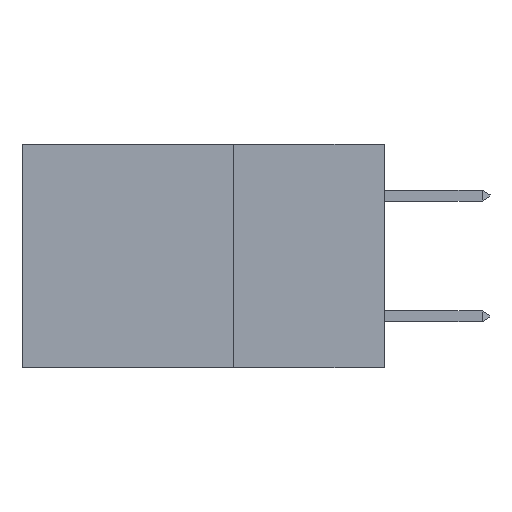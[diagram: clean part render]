
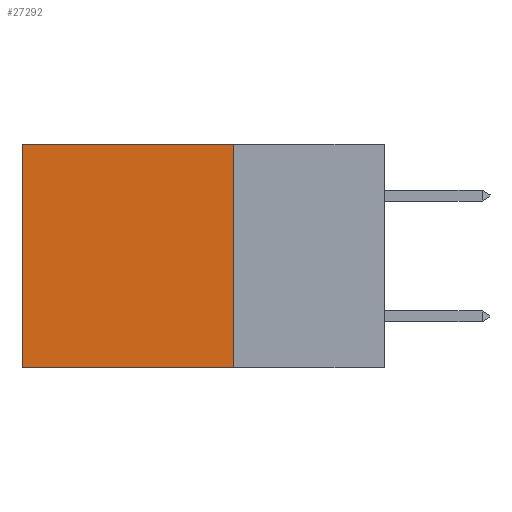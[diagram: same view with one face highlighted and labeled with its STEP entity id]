
A CAD part, left-side view. The second image highlights one B-rep face of the part: STEP entity #27292.
In plain terms, the highlighted planar face has unit normal (-1, 0, 0).
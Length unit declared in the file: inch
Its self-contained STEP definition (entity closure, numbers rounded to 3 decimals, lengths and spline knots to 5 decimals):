
#232 = EDGE_CURVE ( 'NONE', #1115, #25379, #8857, .T. ) ;
#1115 = VERTEX_POINT ( 'NONE', #8701 ) ;
#1706 = DIRECTION ( 'NONE',  ( 0., 0., -1. ) ) ;
#2444 = ORIENTED_EDGE ( 'NONE', *, *, #23544, .F. ) ;
#2747 = CARTESIAN_POINT ( 'NONE',  ( 0.2875, 0.25, -0.37 ) ) ;
#4359 = CARTESIAN_POINT ( 'NONE',  ( 0.2875, 0.25, 0. ) ) ;
#5426 = VERTEX_POINT ( 'NONE', #18399 ) ;
#8701 = CARTESIAN_POINT ( 'NONE',  ( 0.2875, 0.6, 0. ) ) ;
#8857 = LINE ( 'NONE', #19627, #31252 ) ;
#9338 = DIRECTION ( 'NONE',  ( 1., 0., 0. ) ) ;
#9750 = VECTOR ( 'NONE', #28491, 39.37008 ) ;
#13326 = ORIENTED_EDGE ( 'NONE', *, *, #232, .T. ) ;
#13913 = DIRECTION ( 'NONE',  ( 0., 1., 0. ) ) ;
#15936 = EDGE_LOOP ( 'NONE', ( #13326, #2444, #22675, #24786 ) ) ;
#16980 = LINE ( 'NONE', #4359, #9750 ) ;
#18399 = CARTESIAN_POINT ( 'NONE',  ( 0.2875, 0.25, 0. ) ) ;
#19078 = EDGE_CURVE ( 'NONE', #5426, #1115, #28894, .T. ) ;
#19394 = DIRECTION ( 'NONE',  ( 0., 0., -1. ) ) ;
#19627 = CARTESIAN_POINT ( 'NONE',  ( 0.2875, 0.6, 0. ) ) ;
#20746 = EDGE_CURVE ( 'NONE', #5426, #29613, #16980, .T. ) ;
#21754 = VECTOR ( 'NONE', #25723, 39.37008 ) ;
#22392 = PLANE ( 'NONE',  #24016 ) ;
#22675 = ORIENTED_EDGE ( 'NONE', *, *, #20746, .F. ) ;
#22738 = CARTESIAN_POINT ( 'NONE',  ( 0.2875, 0.25, 0. ) ) ;
#23544 = EDGE_CURVE ( 'NONE', #29613, #25379, #27565, .T. ) ;
#24016 = AXIS2_PLACEMENT_3D ( 'NONE', #22738, #9338, #1706 ) ;
#24174 = VECTOR ( 'NONE', #13913, 39.37008 ) ;
#24786 = ORIENTED_EDGE ( 'NONE', *, *, #19078, .T. ) ;
#25379 = VERTEX_POINT ( 'NONE', #27069 ) ;
#25723 = DIRECTION ( 'NONE',  ( 0., 1., 0. ) ) ;
#27069 = CARTESIAN_POINT ( 'NONE',  ( 0.2875, 0.6, -0.37 ) ) ;
#27292 = ADVANCED_FACE ( 'NONE', ( #31078 ), #22392, .F. ) ;
#27565 = LINE ( 'NONE', #2747, #24174 ) ;
#28491 = DIRECTION ( 'NONE',  ( 0., 0., -1. ) ) ;
#28894 = LINE ( 'NONE', #34002, #21754 ) ;
#29613 = VERTEX_POINT ( 'NONE', #31307 ) ;
#31078 = FACE_OUTER_BOUND ( 'NONE', #15936, .T. ) ;
#31252 = VECTOR ( 'NONE', #19394, 39.37008 ) ;
#31307 = CARTESIAN_POINT ( 'NONE',  ( 0.2875, 0.25, -0.37 ) ) ;
#34002 = CARTESIAN_POINT ( 'NONE',  ( 0.2875, 0.25, 0. ) ) ;
